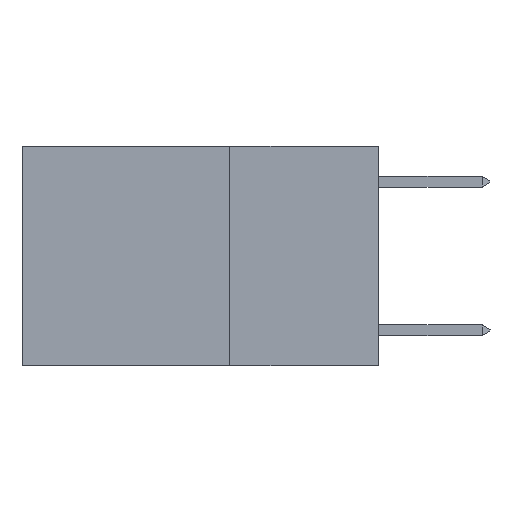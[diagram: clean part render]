
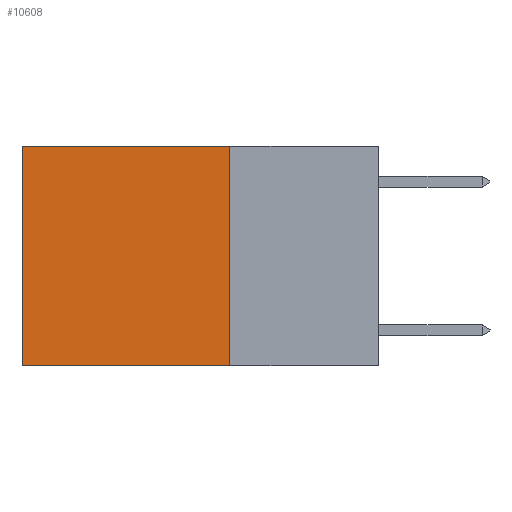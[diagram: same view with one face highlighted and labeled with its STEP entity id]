
A CAD part, left-side view. The second image highlights one B-rep face of the part: STEP entity #10608.
In plain terms, the highlighted planar face has unit normal (-1, 0, 0).
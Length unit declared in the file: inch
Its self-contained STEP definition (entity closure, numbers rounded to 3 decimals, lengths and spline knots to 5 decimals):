
#655 = EDGE_CURVE ( 'NONE', #9433, #21546, #6595, .T. ) ;
#1017 = LINE ( 'NONE', #14053, #20102 ) ;
#1867 = VERTEX_POINT ( 'NONE', #6784 ) ;
#3199 = EDGE_CURVE ( 'NONE', #13827, #1867, #5221, .T. ) ;
#4031 = ORIENTED_EDGE ( 'NONE', *, *, #22608, .T. ) ;
#5175 = VECTOR ( 'NONE', #23559, 39.37008 ) ;
#5221 = LINE ( 'NONE', #9966, #5175 ) ;
#5281 = FACE_OUTER_BOUND ( 'NONE', #19775, .T. ) ;
#5827 = DIRECTION ( 'NONE',  ( 0., 0., -1. ) ) ;
#6170 = CARTESIAN_POINT ( 'NONE',  ( 0.2625, 0.25, 0. ) ) ;
#6285 = VECTOR ( 'NONE', #8082, 39.37008 ) ;
#6595 = LINE ( 'NONE', #9272, #6285 ) ;
#6784 = CARTESIAN_POINT ( 'NONE',  ( 0.2625, 0.6, 0. ) ) ;
#7567 = ORIENTED_EDGE ( 'NONE', *, *, #655, .F. ) ;
#8082 = DIRECTION ( 'NONE',  ( 0., 1., 0. ) ) ;
#9272 = CARTESIAN_POINT ( 'NONE',  ( 0.2625, 0.25, -0.37 ) ) ;
#9433 = VERTEX_POINT ( 'NONE', #9818 ) ;
#9818 = CARTESIAN_POINT ( 'NONE',  ( 0.2625, 0.25, -0.37 ) ) ;
#9966 = CARTESIAN_POINT ( 'NONE',  ( 0.2625, 0.25, 0. ) ) ;
#10608 = ADVANCED_FACE ( 'NONE', ( #5281 ), #17336, .F. ) ;
#10877 = AXIS2_PLACEMENT_3D ( 'NONE', #16936, #16730, #16302 ) ;
#12750 = CARTESIAN_POINT ( 'NONE',  ( 0.2625, 0.25, 0. ) ) ;
#12873 = EDGE_CURVE ( 'NONE', #13827, #9433, #20709, .T. ) ;
#12960 = CARTESIAN_POINT ( 'NONE',  ( 0.2625, 0.6, -0.37 ) ) ;
#13827 = VERTEX_POINT ( 'NONE', #12750 ) ;
#13953 = ORIENTED_EDGE ( 'NONE', *, *, #12873, .F. ) ;
#14053 = CARTESIAN_POINT ( 'NONE',  ( 0.2625, 0.6, 0. ) ) ;
#15294 = ORIENTED_EDGE ( 'NONE', *, *, #3199, .T. ) ;
#16302 = DIRECTION ( 'NONE',  ( 0., 0., -1. ) ) ;
#16730 = DIRECTION ( 'NONE',  ( 1., 0., 0. ) ) ;
#16936 = CARTESIAN_POINT ( 'NONE',  ( 0.2625, 0.25, 0. ) ) ;
#17336 = PLANE ( 'NONE',  #10877 ) ;
#19775 = EDGE_LOOP ( 'NONE', ( #4031, #7567, #13953, #15294 ) ) ;
#20102 = VECTOR ( 'NONE', #21371, 39.37008 ) ;
#20642 = VECTOR ( 'NONE', #5827, 39.37008 ) ;
#20709 = LINE ( 'NONE', #6170, #20642 ) ;
#21371 = DIRECTION ( 'NONE',  ( 0., 0., -1. ) ) ;
#21546 = VERTEX_POINT ( 'NONE', #12960 ) ;
#22608 = EDGE_CURVE ( 'NONE', #1867, #21546, #1017, .T. ) ;
#23559 = DIRECTION ( 'NONE',  ( 0., 1., 0. ) ) ;
